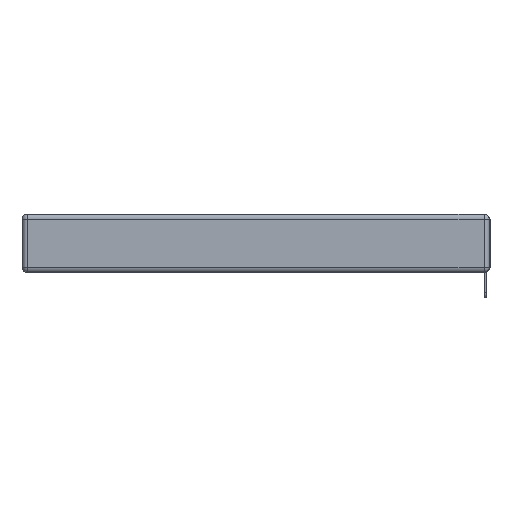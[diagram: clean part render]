
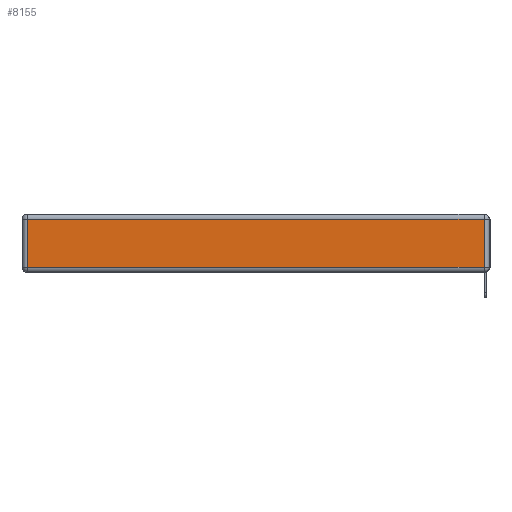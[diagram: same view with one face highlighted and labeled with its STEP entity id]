
A CAD part, left-side view. The second image highlights one B-rep face of the part: STEP entity #8155.
In plain terms, the highlighted planar face has unit normal (-1, 0, 0).
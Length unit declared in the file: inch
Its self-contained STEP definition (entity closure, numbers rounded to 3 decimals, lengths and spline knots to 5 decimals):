
#1095 = ORIENTED_EDGE ( 'NONE', *, *, #2405, .T. ) ;
#1348 = VECTOR ( 'NONE', #21205, 39.37008 ) ;
#1359 = VERTEX_POINT ( 'NONE', #9160 ) ;
#1422 = FACE_OUTER_BOUND ( 'NONE', #3556, .T. ) ;
#1956 = PLANE ( 'NONE',  #19399 ) ;
#2016 = LINE ( 'NONE', #12600, #11409 ) ;
#2037 = DIRECTION ( 'NONE',  ( -1., 0., 0. ) ) ;
#2405 = EDGE_CURVE ( 'NONE', #3088, #8794, #6342, .T. ) ;
#3088 = VERTEX_POINT ( 'NONE', #19181 ) ;
#3556 = EDGE_LOOP ( 'NONE', ( #14989, #1095, #3725, #12804 ) ) ;
#3725 = ORIENTED_EDGE ( 'NONE', *, *, #4321, .T. ) ;
#4321 = EDGE_CURVE ( 'NONE', #8794, #1359, #7435, .T. ) ;
#6342 = LINE ( 'NONE', #22432, #1348 ) ;
#6502 = DIRECTION ( 'NONE',  ( 0., 0., -1. ) ) ;
#7391 = CARTESIAN_POINT ( 'NONE',  ( 0., 2.72, -0.313 ) ) ;
#7435 = LINE ( 'NONE', #16978, #14495 ) ;
#8155 = ADVANCED_FACE ( 'NONE', ( #1422 ), #1956, .T. ) ;
#8794 = VERTEX_POINT ( 'NONE', #23098 ) ;
#9160 = CARTESIAN_POINT ( 'NONE',  ( 0., 2.72, -0.03 ) ) ;
#9200 = VERTEX_POINT ( 'NONE', #7391 ) ;
#10206 = CARTESIAN_POINT ( 'NONE',  ( 0., 2.72, -0.343 ) ) ;
#11229 = EDGE_CURVE ( 'NONE', #1359, #9200, #11234, .T. ) ;
#11234 = LINE ( 'NONE', #10206, #12465 ) ;
#11409 = VECTOR ( 'NONE', #18018, 39.37008 ) ;
#12465 = VECTOR ( 'NONE', #6502, 39.37008 ) ;
#12600 = CARTESIAN_POINT ( 'NONE',  ( 0., 0., -0.313 ) ) ;
#12804 = ORIENTED_EDGE ( 'NONE', *, *, #11229, .T. ) ;
#13450 = DIRECTION ( 'NONE',  ( 0., 1., 0. ) ) ;
#14495 = VECTOR ( 'NONE', #13450, 39.37008 ) ;
#14989 = ORIENTED_EDGE ( 'NONE', *, *, #16667, .T. ) ;
#15185 = DIRECTION ( 'NONE',  ( 0., 0., 1. ) ) ;
#16667 = EDGE_CURVE ( 'NONE', #9200, #3088, #2016, .T. ) ;
#16978 = CARTESIAN_POINT ( 'NONE',  ( 0., 2.75, -0.03 ) ) ;
#18018 = DIRECTION ( 'NONE',  ( 0., -1., 0. ) ) ;
#18873 = CARTESIAN_POINT ( 'NONE',  ( 0., 0., -0.343 ) ) ;
#19181 = CARTESIAN_POINT ( 'NONE',  ( 0., 0.03, -0.313 ) ) ;
#19399 = AXIS2_PLACEMENT_3D ( 'NONE', #18873, #2037, #15185 ) ;
#21205 = DIRECTION ( 'NONE',  ( 0., 0., 1. ) ) ;
#22432 = CARTESIAN_POINT ( 'NONE',  ( 0., 0.03, -0.343 ) ) ;
#23098 = CARTESIAN_POINT ( 'NONE',  ( 0., 0.03, -0.03 ) ) ;
